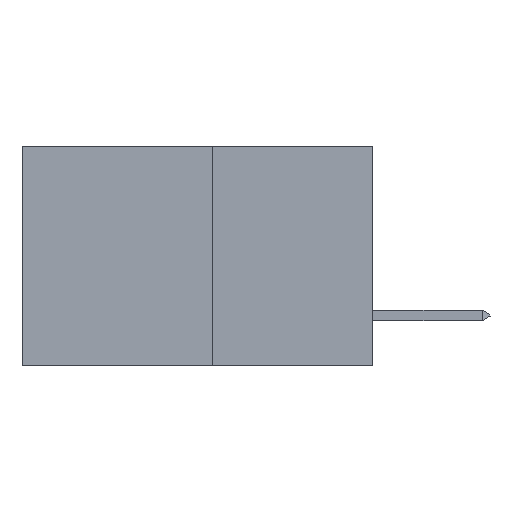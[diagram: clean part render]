
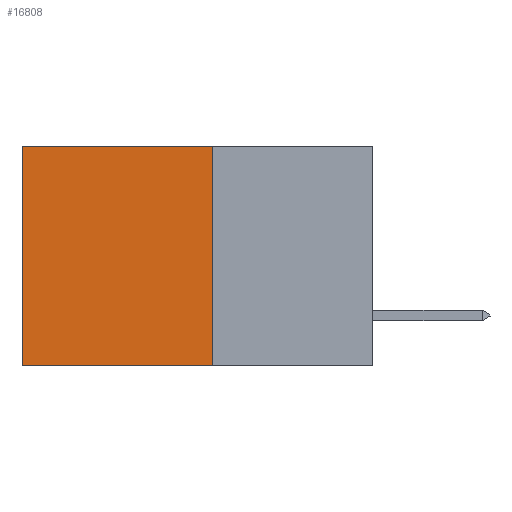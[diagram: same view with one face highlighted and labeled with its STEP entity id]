
A CAD part, left-side view. The second image highlights one B-rep face of the part: STEP entity #16808.
In plain terms, the highlighted planar face has unit normal (-1, 0, 0).
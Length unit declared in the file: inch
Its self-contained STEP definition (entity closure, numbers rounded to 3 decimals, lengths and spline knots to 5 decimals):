
#817 = CARTESIAN_POINT ( 'NONE',  ( 0.277, 0.59, 0. ) ) ;
#1251 = ORIENTED_EDGE ( 'NONE', *, *, #3935, .T. ) ;
#2248 = VERTEX_POINT ( 'NONE', #7082 ) ;
#2289 = EDGE_CURVE ( 'NONE', #8813, #4198, #10688, .T. ) ;
#2887 = AXIS2_PLACEMENT_3D ( 'NONE', #17858, #8169, #17913 ) ;
#3823 = CARTESIAN_POINT ( 'NONE',  ( 0.277, 0.59, -0.37 ) ) ;
#3935 = EDGE_CURVE ( 'NONE', #4198, #13347, #17950, .T. ) ;
#4198 = VERTEX_POINT ( 'NONE', #817 ) ;
#4414 = CARTESIAN_POINT ( 'NONE',  ( 0.277, 0.27, 0. ) ) ;
#5061 = EDGE_CURVE ( 'NONE', #2248, #13347, #17699, .T. ) ;
#5339 = PLANE ( 'NONE',  #2887 ) ;
#6211 = CARTESIAN_POINT ( 'NONE',  ( 0.277, 0.27, 0. ) ) ;
#6433 = VECTOR ( 'NONE', #14894, 39.37008 ) ;
#6876 = LINE ( 'NONE', #7846, #6433 ) ;
#7082 = CARTESIAN_POINT ( 'NONE',  ( 0.277, 0.27, -0.37 ) ) ;
#7846 = CARTESIAN_POINT ( 'NONE',  ( 0.277, 0.27, -0.37 ) ) ;
#8169 = DIRECTION ( 'NONE',  ( 1., 0., 0. ) ) ;
#8813 = VERTEX_POINT ( 'NONE', #4414 ) ;
#9842 = VECTOR ( 'NONE', #17520, 39.37008 ) ;
#10535 = VECTOR ( 'NONE', #16942, 39.37008 ) ;
#10688 = LINE ( 'NONE', #6211, #17661 ) ;
#13347 = VERTEX_POINT ( 'NONE', #14219 ) ;
#13835 = DIRECTION ( 'NONE',  ( 0., 1., 0. ) ) ;
#14085 = ORIENTED_EDGE ( 'NONE', *, *, #2289, .T. ) ;
#14219 = CARTESIAN_POINT ( 'NONE',  ( 0.277, 0.59, -0.37 ) ) ;
#14562 = EDGE_LOOP ( 'NONE', ( #1251, #16292, #15781, #14085 ) ) ;
#14894 = DIRECTION ( 'NONE',  ( 0., 0., -1. ) ) ;
#15781 = ORIENTED_EDGE ( 'NONE', *, *, #17205, .F. ) ;
#16292 = ORIENTED_EDGE ( 'NONE', *, *, #5061, .F. ) ;
#16808 = ADVANCED_FACE ( 'NONE', ( #17589 ), #5339, .F. ) ;
#16942 = DIRECTION ( 'NONE',  ( 0., 0., -1. ) ) ;
#17205 = EDGE_CURVE ( 'NONE', #8813, #2248, #6876, .T. ) ;
#17520 = DIRECTION ( 'NONE',  ( 0., 1., 0. ) ) ;
#17564 = CARTESIAN_POINT ( 'NONE',  ( 0.277, 0.27, -0.37 ) ) ;
#17589 = FACE_OUTER_BOUND ( 'NONE', #14562, .T. ) ;
#17661 = VECTOR ( 'NONE', #13835, 39.37008 ) ;
#17699 = LINE ( 'NONE', #17564, #9842 ) ;
#17858 = CARTESIAN_POINT ( 'NONE',  ( 0.277, 0.27, -0.37 ) ) ;
#17913 = DIRECTION ( 'NONE',  ( 0., 0., -1. ) ) ;
#17950 = LINE ( 'NONE', #3823, #10535 ) ;
